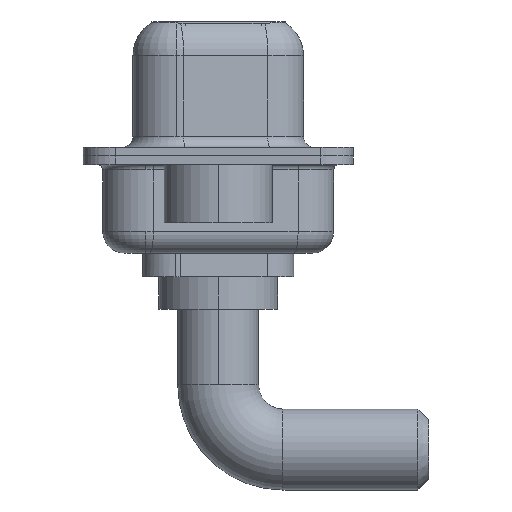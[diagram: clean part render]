
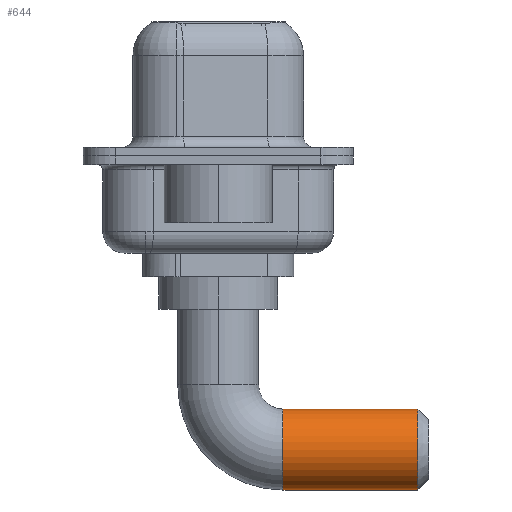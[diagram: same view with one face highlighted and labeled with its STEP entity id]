
A CAD part, left-side view. The second image highlights one B-rep face of the part: STEP entity #644.
In plain terms, the highlighted cylindrical face has radius 1.875 mm (diameter 3.75 mm), a partial arc.
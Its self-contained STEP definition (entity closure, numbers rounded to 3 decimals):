
#17 = DIRECTION ( 'NONE',  ( 0., -1., 0. ) ) ;
#193 = CARTESIAN_POINT ( 'NONE',  ( 0., -3., -4.625 ) ) ;
#206 = CARTESIAN_POINT ( 'NONE',  ( 0., -3., -8.375 ) ) ;
#218 = CARTESIAN_POINT ( 'NONE',  ( 0., -3., -4.625 ) ) ;
#434 = EDGE_CURVE ( 'NONE', #11716, #2618, #7486, .T. ) ;
#644 = ADVANCED_FACE ( 'NONE', ( #1553 ), #2353, .T. ) ;
#692 = DIRECTION ( 'NONE',  ( 0., 0., -1. ) ) ;
#933 = ORIENTED_EDGE ( 'NONE', *, *, #434, .T. ) ;
#1452 = CIRCLE ( 'NONE', #8527, 1.875 ) ;
#1553 = FACE_OUTER_BOUND ( 'NONE', #3029, .T. ) ;
#1668 = VECTOR ( 'NONE', #9541, 1000. ) ;
#1811 = DIRECTION ( 'NONE',  ( 0., -1., 0. ) ) ;
#2353 = CYLINDRICAL_SURFACE ( 'NONE', #4558, 1.875 ) ;
#2618 = VERTEX_POINT ( 'NONE', #3807 ) ;
#3029 = EDGE_LOOP ( 'NONE', ( #5656, #933, #4854, #12011 ) ) ;
#3556 = AXIS2_PLACEMENT_3D ( 'NONE', #9120, #1811, #9307 ) ;
#3807 = CARTESIAN_POINT ( 'NONE',  ( 0., -3., -8.375 ) ) ;
#4558 = AXIS2_PLACEMENT_3D ( 'NONE', #8862, #7077, #11555 ) ;
#4566 = CARTESIAN_POINT ( 'NONE',  ( 0., -9.25, -4.625 ) ) ;
#4854 = ORIENTED_EDGE ( 'NONE', *, *, #9770, .T. ) ;
#5656 = ORIENTED_EDGE ( 'NONE', *, *, #10372, .F. ) ;
#7077 = DIRECTION ( 'NONE',  ( 0., -1., 0. ) ) ;
#7486 = CIRCLE ( 'NONE', #3556, 1.875 ) ;
#7581 = LINE ( 'NONE', #206, #1668 ) ;
#8354 = VERTEX_POINT ( 'NONE', #8758 ) ;
#8527 = AXIS2_PLACEMENT_3D ( 'NONE', #9033, #9219, #692 ) ;
#8758 = CARTESIAN_POINT ( 'NONE',  ( 0., -9.25, -8.375 ) ) ;
#8862 = CARTESIAN_POINT ( 'NONE',  ( 0., -3., -6.5 ) ) ;
#8973 = EDGE_CURVE ( 'NONE', #8354, #8992, #1452, .T. ) ;
#8992 = VERTEX_POINT ( 'NONE', #4566 ) ;
#9033 = CARTESIAN_POINT ( 'NONE',  ( 0., -9.25, -6.5 ) ) ;
#9120 = CARTESIAN_POINT ( 'NONE',  ( 0., -3., -6.5 ) ) ;
#9219 = DIRECTION ( 'NONE',  ( 0., 1., 0. ) ) ;
#9307 = DIRECTION ( 'NONE',  ( -1., 0., 0. ) ) ;
#9541 = DIRECTION ( 'NONE',  ( 0., -1., 0. ) ) ;
#9770 = EDGE_CURVE ( 'NONE', #2618, #8354, #7581, .T. ) ;
#10372 = EDGE_CURVE ( 'NONE', #11716, #8992, #10506, .T. ) ;
#10506 = LINE ( 'NONE', #193, #12075 ) ;
#11555 = DIRECTION ( 'NONE',  ( 0., 0., -1. ) ) ;
#11716 = VERTEX_POINT ( 'NONE', #218 ) ;
#12011 = ORIENTED_EDGE ( 'NONE', *, *, #8973, .T. ) ;
#12075 = VECTOR ( 'NONE', #17, 1000. ) ;
